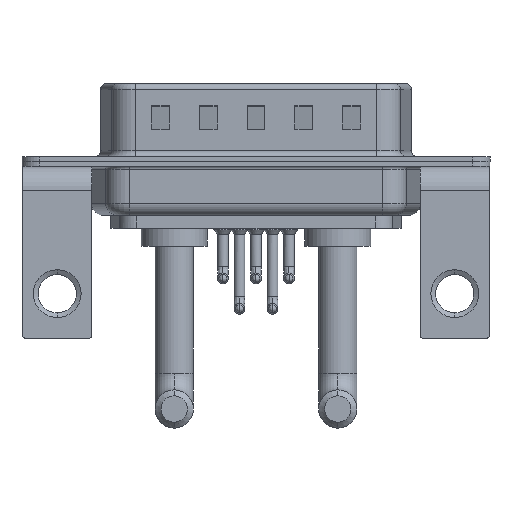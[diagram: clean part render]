
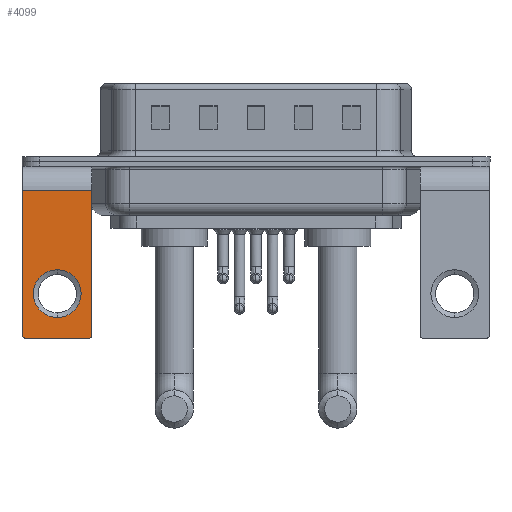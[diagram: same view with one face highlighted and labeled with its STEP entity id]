
A CAD part, front view. The second image highlights one B-rep face of the part: STEP entity #4099.
In plain terms, the highlighted planar face has unit normal (0, -1, 0).
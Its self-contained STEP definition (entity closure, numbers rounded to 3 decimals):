
#170 = CARTESIAN_POINT ( 'NONE',  ( 2.65, -6.25, -14.55 ) ) ;
#1185 = DIRECTION ( 'NONE',  ( 0., 1., 0. ) ) ;
#1391 = DIRECTION ( 'NONE',  ( -1., 0., 0. ) ) ;
#1440 = DIRECTION ( 'NONE',  ( -1., 0., 0. ) ) ;
#1566 = CARTESIAN_POINT ( 'NONE',  ( 2.9, -6.25, -2.4 ) ) ;
#2284 = LINE ( 'NONE', #9033, #5310 ) ;
#2398 = EDGE_CURVE ( 'NONE', #9798, #18953, #18484, .T. ) ;
#2610 = EDGE_LOOP ( 'NONE', ( #9464, #3465 ) ) ;
#2909 = CARTESIAN_POINT ( 'NONE',  ( 2.9, -6.25, -14.55 ) ) ;
#3465 = ORIENTED_EDGE ( 'NONE', *, *, #13489, .T. ) ;
#3480 = VERTEX_POINT ( 'NONE', #2909 ) ;
#3641 = VERTEX_POINT ( 'NONE', #17744 ) ;
#4047 = DIRECTION ( 'NONE',  ( 0., 0., -1. ) ) ;
#4053 = AXIS2_PLACEMENT_3D ( 'NONE', #14858, #18203, #19851 ) ;
#4099 = ADVANCED_FACE ( 'NONE', ( #14777, #19434 ), #4494, .F. ) ;
#4489 = VERTEX_POINT ( 'NONE', #21260 ) ;
#4494 = PLANE ( 'NONE',  #18087 ) ;
#5155 = ORIENTED_EDGE ( 'NONE', *, *, #6251, .F. ) ;
#5310 = VECTOR ( 'NONE', #4047, 1000. ) ;
#5403 = CIRCLE ( 'NONE', #9645, 2. ) ;
#5426 = CARTESIAN_POINT ( 'NONE',  ( -2.9, -6.25, -2.4 ) ) ;
#5494 = VERTEX_POINT ( 'NONE', #14806 ) ;
#5612 = CARTESIAN_POINT ( 'NONE',  ( -2.9, -6.25, -14.55 ) ) ;
#6251 = EDGE_CURVE ( 'NONE', #4489, #3480, #2284, .T. ) ;
#6370 = VECTOR ( 'NONE', #20261, 1000. ) ;
#6626 = ORIENTED_EDGE ( 'NONE', *, *, #6813, .F. ) ;
#6813 = EDGE_CURVE ( 'NONE', #20834, #3641, #18331, .T. ) ;
#6912 = VERTEX_POINT ( 'NONE', #15860 ) ;
#8588 = CARTESIAN_POINT ( 'NONE',  ( 0., -6.25, -11.07 ) ) ;
#9033 = CARTESIAN_POINT ( 'NONE',  ( 2.9, -6.25, -2.4 ) ) ;
#9464 = ORIENTED_EDGE ( 'NONE', *, *, #16114, .T. ) ;
#9501 = DIRECTION ( 'NONE',  ( 0., 0., 1. ) ) ;
#9645 = AXIS2_PLACEMENT_3D ( 'NONE', #8588, #17128, #17227 ) ;
#9798 = VERTEX_POINT ( 'NONE', #14349 ) ;
#10341 = VECTOR ( 'NONE', #1391, 1000. ) ;
#11387 = CARTESIAN_POINT ( 'NONE',  ( 0., -6.25, -11.07 ) ) ;
#11454 = CARTESIAN_POINT ( 'NONE',  ( 2.65, -6.25, -14.8 ) ) ;
#11993 = DIRECTION ( 'NONE',  ( 0., 0., 1. ) ) ;
#12394 = AXIS2_PLACEMENT_3D ( 'NONE', #11387, #16062, #9501 ) ;
#13147 = CIRCLE ( 'NONE', #16361, 0.25 ) ;
#13489 = EDGE_CURVE ( 'NONE', #5494, #6912, #16993, .T. ) ;
#14040 = ORIENTED_EDGE ( 'NONE', *, *, #20974, .T. ) ;
#14349 = CARTESIAN_POINT ( 'NONE',  ( -2.9, -6.25, -2.4 ) ) ;
#14357 = CARTESIAN_POINT ( 'NONE',  ( 2.9, -6.25, -2.4 ) ) ;
#14690 = CARTESIAN_POINT ( 'NONE',  ( 2.9, -6.25, -14.8 ) ) ;
#14777 = FACE_BOUND ( 'NONE', #2610, .T. ) ;
#14806 = CARTESIAN_POINT ( 'NONE',  ( 0., -6.25, -9.07 ) ) ;
#14858 = CARTESIAN_POINT ( 'NONE',  ( -2.65, -6.25, -14.55 ) ) ;
#15323 = DIRECTION ( 'NONE',  ( 0., -1., 0. ) ) ;
#15860 = CARTESIAN_POINT ( 'NONE',  ( 0., -6.25, -13.07 ) ) ;
#16062 = DIRECTION ( 'NONE',  ( 0., 1., 0. ) ) ;
#16114 = EDGE_CURVE ( 'NONE', #6912, #5494, #5403, .T. ) ;
#16361 = AXIS2_PLACEMENT_3D ( 'NONE', #170, #15323, #11993 ) ;
#16993 = CIRCLE ( 'NONE', #12394, 2. ) ;
#17028 = ORIENTED_EDGE ( 'NONE', *, *, #17770, .T. ) ;
#17128 = DIRECTION ( 'NONE',  ( 0., 1., 0. ) ) ;
#17227 = DIRECTION ( 'NONE',  ( 0., 0., 1. ) ) ;
#17744 = CARTESIAN_POINT ( 'NONE',  ( -2.65, -6.25, -14.8 ) ) ;
#17770 = EDGE_CURVE ( 'NONE', #18953, #3641, #21717, .T. ) ;
#17896 = DIRECTION ( 'NONE',  ( 0., 0., 1. ) ) ;
#17938 = ORIENTED_EDGE ( 'NONE', *, *, #2398, .T. ) ;
#18087 = AXIS2_PLACEMENT_3D ( 'NONE', #14357, #1185, #17896 ) ;
#18203 = DIRECTION ( 'NONE',  ( 0., -1., 0. ) ) ;
#18216 = EDGE_LOOP ( 'NONE', ( #17938, #17028, #6626, #14040, #5155, #21512 ) ) ;
#18331 = LINE ( 'NONE', #14690, #10341 ) ;
#18375 = LINE ( 'NONE', #1566, #20223 ) ;
#18484 = LINE ( 'NONE', #5426, #6370 ) ;
#18953 = VERTEX_POINT ( 'NONE', #5612 ) ;
#19434 = FACE_OUTER_BOUND ( 'NONE', #18216, .T. ) ;
#19851 = DIRECTION ( 'NONE',  ( 0., 0., 1. ) ) ;
#20143 = EDGE_CURVE ( 'NONE', #4489, #9798, #18375, .T. ) ;
#20223 = VECTOR ( 'NONE', #1440, 1000. ) ;
#20261 = DIRECTION ( 'NONE',  ( 0., 0., -1. ) ) ;
#20834 = VERTEX_POINT ( 'NONE', #11454 ) ;
#20974 = EDGE_CURVE ( 'NONE', #20834, #3480, #13147, .T. ) ;
#21260 = CARTESIAN_POINT ( 'NONE',  ( 2.9, -6.25, -2.4 ) ) ;
#21512 = ORIENTED_EDGE ( 'NONE', *, *, #20143, .T. ) ;
#21717 = CIRCLE ( 'NONE', #4053, 0.25 ) ;
